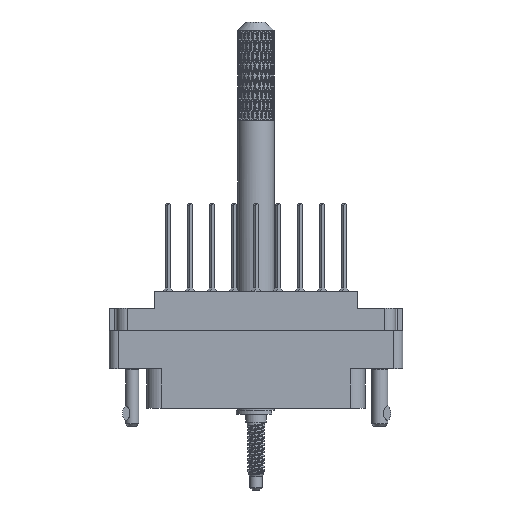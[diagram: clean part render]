
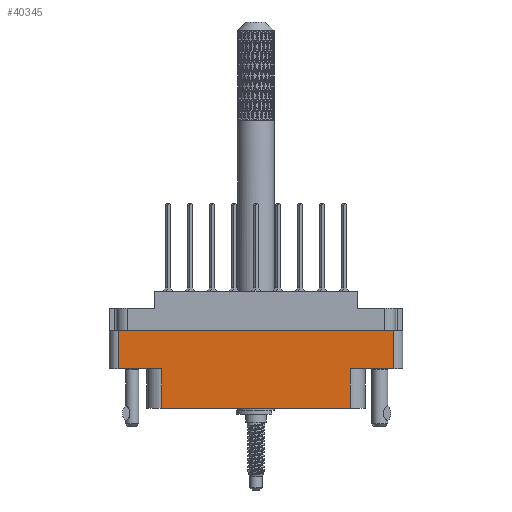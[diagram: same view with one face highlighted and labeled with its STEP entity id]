
A CAD part, front view. The second image highlights one B-rep face of the part: STEP entity #40345.
In plain terms, the highlighted planar face has unit normal (0, -1, 0).
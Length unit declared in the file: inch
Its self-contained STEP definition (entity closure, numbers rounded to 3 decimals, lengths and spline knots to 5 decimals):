
#2259 = CARTESIAN_POINT ( 'NONE',  ( 0., -0.438, -0.529 ) ) ;
#2339 = VECTOR ( 'NONE', #55244, 39.37008 ) ;
#2839 = CARTESIAN_POINT ( 'NONE',  ( -0.938, -0.438, -0.798 ) ) ;
#9230 = VECTOR ( 'NONE', #108834, 39.37008 ) ;
#9414 = EDGE_CURVE ( 'NONE', #106633, #87211, #16477, .T. ) ;
#12126 = ORIENTED_EDGE ( 'NONE', *, *, #59261, .T. ) ;
#13066 = LINE ( 'NONE', #50837, #61552 ) ;
#15148 = DIRECTION ( 'NONE',  ( 0., 0., -1. ) ) ;
#16477 = LINE ( 'NONE', #2259, #87907 ) ;
#17330 = LINE ( 'NONE', #108967, #41619 ) ;
#18998 = EDGE_CURVE ( 'NONE', #77524, #87442, #13066, .T. ) ;
#20158 = AXIS2_PLACEMENT_3D ( 'NONE', #66741, #58067, #15148 ) ;
#20263 = LINE ( 'NONE', #47171, #92941 ) ;
#20471 = DIRECTION ( 'NONE',  ( 0., 0., 1. ) ) ;
#21869 = DIRECTION ( 'NONE',  ( 0., 0., 1. ) ) ;
#23378 = ORIENTED_EDGE ( 'NONE', *, *, #59692, .T. ) ;
#23553 = VERTEX_POINT ( 'NONE', #40269 ) ;
#25121 = ORIENTED_EDGE ( 'NONE', *, *, #83243, .T. ) ;
#29837 = VECTOR ( 'NONE', #20471, 39.37008 ) ;
#32041 = LINE ( 'NONE', #65203, #9230 ) ;
#34636 = VERTEX_POINT ( 'NONE', #78911 ) ;
#35202 = CARTESIAN_POINT ( 'NONE',  ( -0.938, -0.438, -0.268 ) ) ;
#37517 = EDGE_CURVE ( 'NONE', #79084, #23553, #60838, .T. ) ;
#39279 = VECTOR ( 'NONE', #61021, 39.37008 ) ;
#40269 = CARTESIAN_POINT ( 'NONE',  ( 0.938, -0.438, -0.268 ) ) ;
#40345 = ADVANCED_FACE ( 'NONE', ( #103514 ), #42244, .T. ) ;
#41619 = VECTOR ( 'NONE', #100668, 39.37008 ) ;
#42244 = PLANE ( 'NONE',  #20158 ) ;
#43582 = CARTESIAN_POINT ( 'NONE',  ( 0.938, -0.438, -0.529 ) ) ;
#46002 = ORIENTED_EDGE ( 'NONE', *, *, #9414, .F. ) ;
#46723 = EDGE_CURVE ( 'NONE', #87211, #109679, #65595, .T. ) ;
#47171 = CARTESIAN_POINT ( 'NONE',  ( 0.938, -0.438, -0.798 ) ) ;
#47458 = LINE ( 'NONE', #2839, #29837 ) ;
#50837 = CARTESIAN_POINT ( 'NONE',  ( -0.644, -0.438, -0.529 ) ) ;
#55244 = DIRECTION ( 'NONE',  ( 0., 0., -1. ) ) ;
#57802 = ORIENTED_EDGE ( 'NONE', *, *, #72174, .F. ) ;
#58067 = DIRECTION ( 'NONE',  ( 0., -1., 0. ) ) ;
#59261 = EDGE_CURVE ( 'NONE', #87442, #109679, #17330, .T. ) ;
#59692 = EDGE_CURVE ( 'NONE', #34636, #77524, #32041, .T. ) ;
#60838 = LINE ( 'NONE', #103934, #39279 ) ;
#61021 = DIRECTION ( 'NONE',  ( 1., 0., 0. ) ) ;
#61552 = VECTOR ( 'NONE', #111020, 39.37008 ) ;
#63202 = DIRECTION ( 'NONE',  ( -1., 0., 0. ) ) ;
#65203 = CARTESIAN_POINT ( 'NONE',  ( 0., -0.438, -0.529 ) ) ;
#65595 = LINE ( 'NONE', #80767, #2339 ) ;
#66122 = ORIENTED_EDGE ( 'NONE', *, *, #46723, .F. ) ;
#66741 = CARTESIAN_POINT ( 'NONE',  ( -0.938, -0.438, -0.798 ) ) ;
#68601 = CARTESIAN_POINT ( 'NONE',  ( -0.644, -0.438, -0.798 ) ) ;
#72174 = EDGE_CURVE ( 'NONE', #34636, #79084, #47458, .T. ) ;
#73186 = EDGE_LOOP ( 'NONE', ( #105484, #12126, #66122, #46002, #25121, #95915, #57802, #23378 ) ) ;
#77524 = VERTEX_POINT ( 'NONE', #95018 ) ;
#78911 = CARTESIAN_POINT ( 'NONE',  ( -0.938, -0.438, -0.529 ) ) ;
#79084 = VERTEX_POINT ( 'NONE', #35202 ) ;
#80767 = CARTESIAN_POINT ( 'NONE',  ( 0.644, -0.438, -0.529 ) ) ;
#81912 = CARTESIAN_POINT ( 'NONE',  ( 0.644, -0.438, -0.798 ) ) ;
#83243 = EDGE_CURVE ( 'NONE', #106633, #23553, #20263, .T. ) ;
#87211 = VERTEX_POINT ( 'NONE', #99136 ) ;
#87442 = VERTEX_POINT ( 'NONE', #68601 ) ;
#87907 = VECTOR ( 'NONE', #63202, 39.37008 ) ;
#92941 = VECTOR ( 'NONE', #21869, 39.37008 ) ;
#95018 = CARTESIAN_POINT ( 'NONE',  ( -0.644, -0.438, -0.529 ) ) ;
#95915 = ORIENTED_EDGE ( 'NONE', *, *, #37517, .F. ) ;
#99136 = CARTESIAN_POINT ( 'NONE',  ( 0.644, -0.438, -0.529 ) ) ;
#100668 = DIRECTION ( 'NONE',  ( 1., 0., 0. ) ) ;
#103514 = FACE_OUTER_BOUND ( 'NONE', #73186, .T. ) ;
#103934 = CARTESIAN_POINT ( 'NONE',  ( -1., -0.438, -0.268 ) ) ;
#105484 = ORIENTED_EDGE ( 'NONE', *, *, #18998, .T. ) ;
#106633 = VERTEX_POINT ( 'NONE', #43582 ) ;
#108834 = DIRECTION ( 'NONE',  ( 1., 0., 0. ) ) ;
#108967 = CARTESIAN_POINT ( 'NONE',  ( -0.938, -0.438, -0.798 ) ) ;
#109679 = VERTEX_POINT ( 'NONE', #81912 ) ;
#111020 = DIRECTION ( 'NONE',  ( 0., 0., -1. ) ) ;
